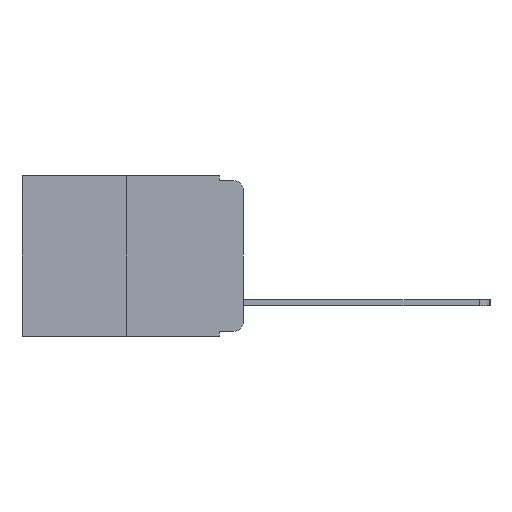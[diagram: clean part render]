
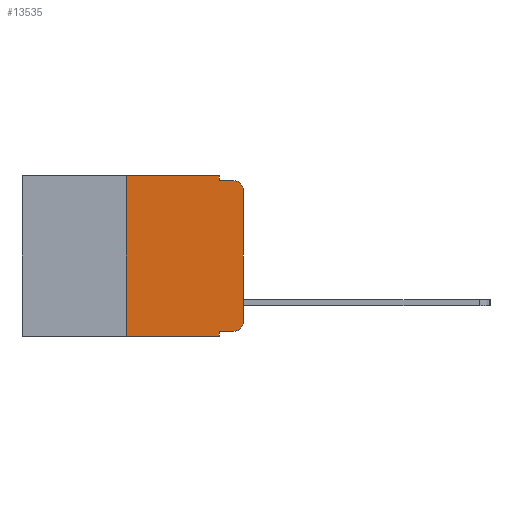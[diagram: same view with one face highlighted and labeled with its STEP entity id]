
A CAD part, left-side view. The second image highlights one B-rep face of the part: STEP entity #13535.
In plain terms, the highlighted planar face has unit normal (-1, 0, 0).
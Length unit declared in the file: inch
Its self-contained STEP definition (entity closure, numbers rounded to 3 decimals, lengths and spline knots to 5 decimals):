
#220 = EDGE_CURVE ( 'NONE', #11477, #9178, #17650, .T. ) ;
#378 = EDGE_CURVE ( 'NONE', #10399, #11477, #18449, .T. ) ;
#1036 = DIRECTION ( 'NONE',  ( 0., 0., -1. ) ) ;
#1126 = CARTESIAN_POINT ( 'NONE',  ( 0., 0.25, 0. ) ) ;
#1445 = EDGE_CURVE ( 'NONE', #10399, #10890, #14775, .T. ) ;
#2409 = CARTESIAN_POINT ( 'NONE',  ( 0., 0.051, -0.333 ) ) ;
#2996 = EDGE_LOOP ( 'NONE', ( #4133, #14130, #3609, #20331, #12030, #12584, #11480, #9906, #18496, #3349 ) ) ;
#2997 = CARTESIAN_POINT ( 'NONE',  ( 0., 0.051, 0. ) ) ;
#3349 = ORIENTED_EDGE ( 'NONE', *, *, #220, .T. ) ;
#3609 = ORIENTED_EDGE ( 'NONE', *, *, #5945, .F. ) ;
#3622 = EDGE_CURVE ( 'NONE', #13404, #20417, #3889, .T. ) ;
#3889 = LINE ( 'NONE', #18797, #12315 ) ;
#4059 = DIRECTION ( 'NONE',  ( 0., 0., -1. ) ) ;
#4133 = ORIENTED_EDGE ( 'NONE', *, *, #9334, .T. ) ;
#4143 = CARTESIAN_POINT ( 'NONE',  ( 0., 0., 0. ) ) ;
#5681 = AXIS2_PLACEMENT_3D ( 'NONE', #13780, #7064, #4059 ) ;
#5770 = VECTOR ( 'NONE', #9216, 39.37008 ) ;
#5794 = CARTESIAN_POINT ( 'NONE',  ( 0., 0.473, -0.343 ) ) ;
#5945 = EDGE_CURVE ( 'NONE', #20417, #6240, #6337, .T. ) ;
#6031 = EDGE_CURVE ( 'NONE', #6479, #11399, #17499, .T. ) ;
#6093 = CARTESIAN_POINT ( 'NONE',  ( 0., 0.051, -0.343 ) ) ;
#6240 = VERTEX_POINT ( 'NONE', #16176 ) ;
#6337 = LINE ( 'NONE', #12116, #10245 ) ;
#6380 = EDGE_CURVE ( 'NONE', #11399, #13404, #14672, .T. ) ;
#6479 = VERTEX_POINT ( 'NONE', #10705 ) ;
#6569 = CARTESIAN_POINT ( 'NONE',  ( 0., 0.051, 0. ) ) ;
#7064 = DIRECTION ( 'NONE',  ( -1., 0., 0. ) ) ;
#7228 = VECTOR ( 'NONE', #15855, 39.37008 ) ;
#7704 = CARTESIAN_POINT ( 'NONE',  ( 0., 0.02, -0.333 ) ) ;
#8517 = DIRECTION ( 'NONE',  ( 0., 0., 1. ) ) ;
#8531 = EDGE_CURVE ( 'NONE', #15269, #6240, #16112, .T. ) ;
#8659 = CARTESIAN_POINT ( 'NONE',  ( 0., 0.02, -0.03 ) ) ;
#9015 = DIRECTION ( 'NONE',  ( 0., 0., -1. ) ) ;
#9178 = VERTEX_POINT ( 'NONE', #20364 ) ;
#9196 = CARTESIAN_POINT ( 'NONE',  ( 0., 0.473, 0. ) ) ;
#9216 = DIRECTION ( 'NONE',  ( 0., -1., 0. ) ) ;
#9334 = EDGE_CURVE ( 'NONE', #9178, #15269, #19993, .T. ) ;
#9906 = ORIENTED_EDGE ( 'NONE', *, *, #1445, .F. ) ;
#10245 = VECTOR ( 'NONE', #19695, 39.37008 ) ;
#10290 = DIRECTION ( 'NONE',  ( 0., 0., -1. ) ) ;
#10297 = VECTOR ( 'NONE', #15794, 39.37008 ) ;
#10399 = VERTEX_POINT ( 'NONE', #2409 ) ;
#10705 = CARTESIAN_POINT ( 'NONE',  ( 0., 0.25, -0.343 ) ) ;
#10759 = EDGE_CURVE ( 'NONE', #6479, #10890, #18629, .T. ) ;
#10890 = VERTEX_POINT ( 'NONE', #6093 ) ;
#11399 = VERTEX_POINT ( 'NONE', #19115 ) ;
#11477 = VERTEX_POINT ( 'NONE', #7704 ) ;
#11480 = ORIENTED_EDGE ( 'NONE', *, *, #10759, .T. ) ;
#12030 = ORIENTED_EDGE ( 'NONE', *, *, #6380, .F. ) ;
#12116 = CARTESIAN_POINT ( 'NONE',  ( 0., 0.051, -0.01 ) ) ;
#12315 = VECTOR ( 'NONE', #17173, 39.37008 ) ;
#12355 = CARTESIAN_POINT ( 'NONE',  ( 0., 0., -0.03 ) ) ;
#12584 = ORIENTED_EDGE ( 'NONE', *, *, #6031, .F. ) ;
#13137 = VECTOR ( 'NONE', #8517, 39.37008 ) ;
#13404 = VERTEX_POINT ( 'NONE', #2997 ) ;
#13535 = ADVANCED_FACE ( 'NONE', ( #21491 ), #20544, .F. ) ;
#13716 = CARTESIAN_POINT ( 'NONE',  ( 0., 0.051, -0.01 ) ) ;
#13780 = CARTESIAN_POINT ( 'NONE',  ( 0., 0.02, -0.313 ) ) ;
#14130 = ORIENTED_EDGE ( 'NONE', *, *, #8531, .T. ) ;
#14256 = VECTOR ( 'NONE', #1036, 39.37008 ) ;
#14672 = LINE ( 'NONE', #9196, #5770 ) ;
#14775 = LINE ( 'NONE', #6569, #14256 ) ;
#15269 = VERTEX_POINT ( 'NONE', #12355 ) ;
#15614 = CARTESIAN_POINT ( 'NONE',  ( 0., 0.473, 0. ) ) ;
#15794 = DIRECTION ( 'NONE',  ( 0., -1., 0. ) ) ;
#15855 = DIRECTION ( 'NONE',  ( 0., 0., 1. ) ) ;
#16112 = CIRCLE ( 'NONE', #18644, 0.02 ) ;
#16176 = CARTESIAN_POINT ( 'NONE',  ( 0., 0.02, -0.01 ) ) ;
#17173 = DIRECTION ( 'NONE',  ( 0., 0., -1. ) ) ;
#17499 = LINE ( 'NONE', #1126, #13137 ) ;
#17650 = CIRCLE ( 'NONE', #5681, 0.02 ) ;
#17922 = VECTOR ( 'NONE', #20660, 39.37008 ) ;
#18449 = LINE ( 'NONE', #20683, #17922 ) ;
#18496 = ORIENTED_EDGE ( 'NONE', *, *, #378, .T. ) ;
#18629 = LINE ( 'NONE', #5794, #10297 ) ;
#18644 = AXIS2_PLACEMENT_3D ( 'NONE', #8659, #20254, #10290 ) ;
#18797 = CARTESIAN_POINT ( 'NONE',  ( 0., 0.051, 0. ) ) ;
#18954 = DIRECTION ( 'NONE',  ( 1., 0., 0. ) ) ;
#19115 = CARTESIAN_POINT ( 'NONE',  ( 0., 0.25, 0. ) ) ;
#19695 = DIRECTION ( 'NONE',  ( 0., -1., 0. ) ) ;
#19993 = LINE ( 'NONE', #4143, #7228 ) ;
#20254 = DIRECTION ( 'NONE',  ( -1., 0., 0. ) ) ;
#20331 = ORIENTED_EDGE ( 'NONE', *, *, #3622, .F. ) ;
#20364 = CARTESIAN_POINT ( 'NONE',  ( 0., 0., -0.313 ) ) ;
#20417 = VERTEX_POINT ( 'NONE', #13716 ) ;
#20544 = PLANE ( 'NONE',  #20808 ) ;
#20660 = DIRECTION ( 'NONE',  ( 0., -1., 0. ) ) ;
#20683 = CARTESIAN_POINT ( 'NONE',  ( 0., 0.051, -0.333 ) ) ;
#20808 = AXIS2_PLACEMENT_3D ( 'NONE', #15614, #18954, #9015 ) ;
#21491 = FACE_OUTER_BOUND ( 'NONE', #2996, .T. ) ;
